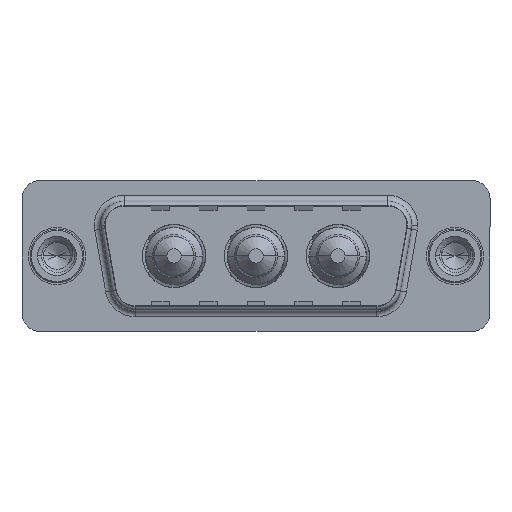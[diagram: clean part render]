
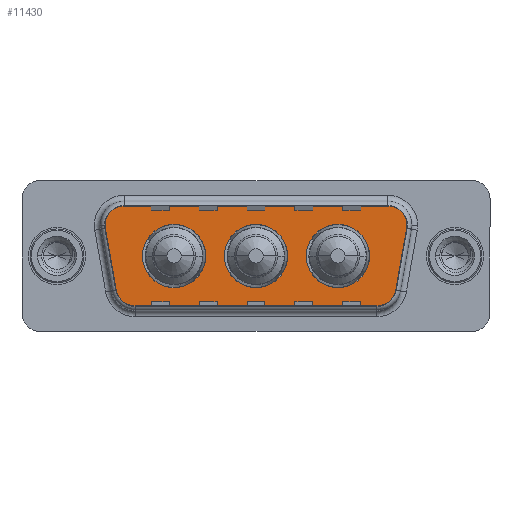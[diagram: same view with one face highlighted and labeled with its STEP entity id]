
A CAD part, top view. The second image highlights one B-rep face of the part: STEP entity #11430.
In plain terms, the highlighted planar face has unit normal (0, 0, 1).
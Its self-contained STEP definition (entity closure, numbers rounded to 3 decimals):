
#103 = VERTEX_POINT ( 'NONE', #378 ) ;
#166 = VERTEX_POINT ( 'NONE', #1659 ) ;
#203 = CARTESIAN_POINT ( 'NONE',  ( 16.65, 0., 0. ) ) ;
#204 = ORIENTED_EDGE ( 'NONE', *, *, #3101, .F. ) ;
#333 = CIRCLE ( 'NONE', #14607, 2.65 ) ;
#378 = CARTESIAN_POINT ( 'NONE',  ( 29.889, 2.9, 0. ) ) ;
#380 = VERTEX_POINT ( 'NONE', #7443 ) ;
#388 = LINE ( 'NONE', #12523, #9387 ) ;
#429 = AXIS2_PLACEMENT_3D ( 'NONE', #5937, #13932, #7087 ) ;
#430 = CIRCLE ( 'NONE', #7367, 2.65 ) ;
#561 = ORIENTED_EDGE ( 'NONE', *, *, #836, .F. ) ;
#836 = EDGE_CURVE ( 'NONE', #380, #11405, #6237, .T. ) ;
#867 = CIRCLE ( 'NONE', #3361, 2.65 ) ;
#938 = EDGE_CURVE ( 'NONE', #3575, #14402, #1811, .T. ) ;
#942 = CARTESIAN_POINT ( 'NONE',  ( 3.441, 2.553, 0. ) ) ;
#986 = CARTESIAN_POINT ( 'NONE',  ( 26.866, -2.9, 0. ) ) ;
#991 = DIRECTION ( 'NONE',  ( 0., 0., 1. ) ) ;
#1006 = CIRCLE ( 'NONE', #9244, 2.65 ) ;
#1277 = DIRECTION ( 'NONE',  ( 1., 0., 0. ) ) ;
#1309 = DIRECTION ( 'NONE',  ( 0.174, -0.985, 0. ) ) ;
#1363 = DIRECTION ( 'NONE',  ( 1., 0., 0. ) ) ;
#1579 = ORIENTED_EDGE ( 'NONE', *, *, #938, .T. ) ;
#1659 = CARTESIAN_POINT ( 'NONE',  ( 19.3, 0., 0. ) ) ;
#1811 = LINE ( 'NONE', #7647, #13191 ) ;
#2110 = DIRECTION ( 'NONE',  ( 0., 0., 1. ) ) ;
#2247 = EDGE_CURVE ( 'NONE', #9616, #3575, #11717, .T. ) ;
#2433 = VERTEX_POINT ( 'NONE', #6880 ) ;
#2488 = AXIS2_PLACEMENT_3D ( 'NONE', #986, #2110, #10003 ) ;
#2741 = ORIENTED_EDGE ( 'NONE', *, *, #8954, .T. ) ;
#2803 = CIRCLE ( 'NONE', #7224, 2. ) ;
#2817 = EDGE_LOOP ( 'NONE', ( #561, #14297 ) ) ;
#3101 = EDGE_CURVE ( 'NONE', #6075, #13467, #5824, .T. ) ;
#3361 = AXIS2_PLACEMENT_3D ( 'NONE', #203, #8092, #1363 ) ;
#3406 = CIRCLE ( 'NONE', #4661, 2. ) ;
#3575 = VERTEX_POINT ( 'NONE', #10072 ) ;
#3636 = DIRECTION ( 'NONE',  ( 0., 0., 1. ) ) ;
#3821 = ORIENTED_EDGE ( 'NONE', *, *, #10178, .T. ) ;
#3835 = CARTESIAN_POINT ( 'NONE',  ( 26.15, 0., 0. ) ) ;
#3862 = LINE ( 'NONE', #10329, #9684 ) ;
#3863 = CARTESIAN_POINT ( 'NONE',  ( 14., 0., 0. ) ) ;
#4349 = CARTESIAN_POINT ( 'NONE',  ( 7.15, 0., 0. ) ) ;
#4410 = EDGE_LOOP ( 'NONE', ( #204, #10141 ) ) ;
#4448 = EDGE_CURVE ( 'NONE', #12923, #7111, #2803, .T. ) ;
#4583 = DIRECTION ( 'NONE',  ( 0.174, 0.985, 0. ) ) ;
#4638 = DIRECTION ( 'NONE',  ( 0., 0., 1. ) ) ;
#4652 = CARTESIAN_POINT ( 'NONE',  ( 28.836, -3.247, 0. ) ) ;
#4661 = AXIS2_PLACEMENT_3D ( 'NONE', #11413, #4638, #12577 ) ;
#4729 = VERTEX_POINT ( 'NONE', #5823 ) ;
#4820 = DIRECTION ( 'NONE',  ( 0., 0., 1. ) ) ;
#5222 = ORIENTED_EDGE ( 'NONE', *, *, #4448, .T. ) ;
#5492 = ORIENTED_EDGE ( 'NONE', *, *, #12227, .F. ) ;
#5501 = LINE ( 'NONE', #13338, #8150 ) ;
#5823 = CARTESIAN_POINT ( 'NONE',  ( 29.859, 2.553, 0. ) ) ;
#5824 = CIRCLE ( 'NONE', #11785, 2.65 ) ;
#5937 = CARTESIAN_POINT ( 'NONE',  ( 27.889, 2.9, 0. ) ) ;
#6075 = VERTEX_POINT ( 'NONE', #3835 ) ;
#6237 = CIRCLE ( 'NONE', #6435, 2.65 ) ;
#6286 = VERTEX_POINT ( 'NONE', #3863 ) ;
#6430 = CIRCLE ( 'NONE', #9067, 2. ) ;
#6435 = AXIS2_PLACEMENT_3D ( 'NONE', #7254, #9954, #7124 ) ;
#6441 = CARTESIAN_POINT ( 'NONE',  ( 9.8, 0., 0. ) ) ;
#6507 = DIRECTION ( 'NONE',  ( -1., 0., 0. ) ) ;
#6655 = ORIENTED_EDGE ( 'NONE', *, *, #13512, .T. ) ;
#6880 = CARTESIAN_POINT ( 'NONE',  ( 27.889, 4.9, 0. ) ) ;
#6899 = FACE_BOUND ( 'NONE', #12753, .T. ) ;
#7061 = CARTESIAN_POINT ( 'NONE',  ( 4.464, -3.247, 0. ) ) ;
#7087 = DIRECTION ( 'NONE',  ( -1., 0., 0. ) ) ;
#7111 = VERTEX_POINT ( 'NONE', #942 ) ;
#7124 = DIRECTION ( 'NONE',  ( 1., 0., 0. ) ) ;
#7143 = EDGE_CURVE ( 'NONE', #6286, #166, #1006, .T. ) ;
#7224 = AXIS2_PLACEMENT_3D ( 'NONE', #11257, #11207, #11157 ) ;
#7254 = CARTESIAN_POINT ( 'NONE',  ( 9.8, 0., 0. ) ) ;
#7367 = AXIS2_PLACEMENT_3D ( 'NONE', #11610, #4820, #12775 ) ;
#7443 = CARTESIAN_POINT ( 'NONE',  ( 12.45, 0., 0. ) ) ;
#7564 = DIRECTION ( 'NONE',  ( 1., 0., 0. ) ) ;
#7647 = CARTESIAN_POINT ( 'NONE',  ( 6.434, -4.9, 0. ) ) ;
#7742 = PLANE ( 'NONE',  #2488 ) ;
#7745 = CARTESIAN_POINT ( 'NONE',  ( 16.65, 0., 0. ) ) ;
#8045 = AXIS2_PLACEMENT_3D ( 'NONE', #8888, #10400, #11605 ) ;
#8092 = DIRECTION ( 'NONE',  ( 0., 0., 1. ) ) ;
#8150 = VECTOR ( 'NONE', #6507, 1000. ) ;
#8243 = DIRECTION ( 'NONE',  ( 0., 0., 1. ) ) ;
#8264 = ORIENTED_EDGE ( 'NONE', *, *, #7143, .F. ) ;
#8442 = EDGE_CURVE ( 'NONE', #13467, #6075, #430, .T. ) ;
#8850 = DIRECTION ( 'NONE',  ( 1., 0., 0. ) ) ;
#8888 = CARTESIAN_POINT ( 'NONE',  ( 6.434, -2.9, 0. ) ) ;
#8954 = EDGE_CURVE ( 'NONE', #14402, #14713, #6430, .T. ) ;
#9067 = AXIS2_PLACEMENT_3D ( 'NONE', #10394, #3636, #11553 ) ;
#9244 = AXIS2_PLACEMENT_3D ( 'NONE', #7745, #991, #8850 ) ;
#9269 = CARTESIAN_POINT ( 'NONE',  ( 5.411, 4.9, 0. ) ) ;
#9387 = VECTOR ( 'NONE', #4583, 1000. ) ;
#9518 = FACE_OUTER_BOUND ( 'NONE', #12945, .T. ) ;
#9616 = VERTEX_POINT ( 'NONE', #7061 ) ;
#9684 = VECTOR ( 'NONE', #1309, 1000. ) ;
#9881 = FACE_BOUND ( 'NONE', #2817, .T. ) ;
#9921 = EDGE_CURVE ( 'NONE', #2433, #12923, #5501, .T. ) ;
#9954 = DIRECTION ( 'NONE',  ( 0., 0., 1. ) ) ;
#10003 = DIRECTION ( 'NONE',  ( 1., 0., 0. ) ) ;
#10072 = CARTESIAN_POINT ( 'NONE',  ( 6.434, -4.9, 0. ) ) ;
#10133 = EDGE_CURVE ( 'NONE', #14713, #4729, #388, .T. ) ;
#10141 = ORIENTED_EDGE ( 'NONE', *, *, #8442, .F. ) ;
#10178 = EDGE_CURVE ( 'NONE', #4729, #103, #3406, .T. ) ;
#10286 = ORIENTED_EDGE ( 'NONE', *, *, #10133, .T. ) ;
#10329 = CARTESIAN_POINT ( 'NONE',  ( 3.441, 2.553, 0. ) ) ;
#10394 = CARTESIAN_POINT ( 'NONE',  ( 26.866, -2.9, 0. ) ) ;
#10400 = DIRECTION ( 'NONE',  ( 0., 0., 1. ) ) ;
#10459 = ORIENTED_EDGE ( 'NONE', *, *, #2247, .T. ) ;
#11157 = DIRECTION ( 'NONE',  ( 1., 0., 0. ) ) ;
#11207 = DIRECTION ( 'NONE',  ( 0., 0., 1. ) ) ;
#11257 = CARTESIAN_POINT ( 'NONE',  ( 5.411, 2.9, 0. ) ) ;
#11304 = DIRECTION ( 'NONE',  ( 1., 0., 0. ) ) ;
#11344 = ORIENTED_EDGE ( 'NONE', *, *, #9921, .T. ) ;
#11405 = VERTEX_POINT ( 'NONE', #4349 ) ;
#11413 = CARTESIAN_POINT ( 'NONE',  ( 27.889, 2.9, 0. ) ) ;
#11430 = ADVANCED_FACE ( 'NONE', ( #6899, #12604, #9881, #9518 ), #7742, .T. ) ;
#11553 = DIRECTION ( 'NONE',  ( 1., 0., 0. ) ) ;
#11605 = DIRECTION ( 'NONE',  ( -1., 0., 0. ) ) ;
#11610 = CARTESIAN_POINT ( 'NONE',  ( 23.5, 0., 0. ) ) ;
#11717 = CIRCLE ( 'NONE', #8045, 2. ) ;
#11785 = AXIS2_PLACEMENT_3D ( 'NONE', #14525, #8243, #11304 ) ;
#11936 = EDGE_CURVE ( 'NONE', #11405, #380, #333, .T. ) ;
#12221 = EDGE_CURVE ( 'NONE', #7111, #9616, #3862, .T. ) ;
#12227 = EDGE_CURVE ( 'NONE', #166, #6286, #867, .T. ) ;
#12523 = CARTESIAN_POINT ( 'NONE',  ( 29.859, 2.553, 0. ) ) ;
#12577 = DIRECTION ( 'NONE',  ( -1., 0., 0. ) ) ;
#12604 = FACE_BOUND ( 'NONE', #4410, .T. ) ;
#12753 = EDGE_LOOP ( 'NONE', ( #5492, #8264 ) ) ;
#12775 = DIRECTION ( 'NONE',  ( 1., 0., 0. ) ) ;
#12923 = VERTEX_POINT ( 'NONE', #9269 ) ;
#12945 = EDGE_LOOP ( 'NONE', ( #2741, #10286, #3821, #6655, #11344, #5222, #14018, #10459, #1579 ) ) ;
#13191 = VECTOR ( 'NONE', #1277, 1000. ) ;
#13197 = CARTESIAN_POINT ( 'NONE',  ( 26.866, -4.9, 0. ) ) ;
#13338 = CARTESIAN_POINT ( 'NONE',  ( 5.411, 4.9, 0. ) ) ;
#13467 = VERTEX_POINT ( 'NONE', #13737 ) ;
#13512 = EDGE_CURVE ( 'NONE', #103, #2433, #14007, .T. ) ;
#13737 = CARTESIAN_POINT ( 'NONE',  ( 20.85, 0., 0. ) ) ;
#13932 = DIRECTION ( 'NONE',  ( 0., 0., 1. ) ) ;
#14007 = CIRCLE ( 'NONE', #429, 2. ) ;
#14018 = ORIENTED_EDGE ( 'NONE', *, *, #12221, .T. ) ;
#14297 = ORIENTED_EDGE ( 'NONE', *, *, #11936, .F. ) ;
#14402 = VERTEX_POINT ( 'NONE', #13197 ) ;
#14439 = DIRECTION ( 'NONE',  ( 0., 0., 1. ) ) ;
#14525 = CARTESIAN_POINT ( 'NONE',  ( 23.5, 0., 0. ) ) ;
#14607 = AXIS2_PLACEMENT_3D ( 'NONE', #6441, #14439, #7564 ) ;
#14713 = VERTEX_POINT ( 'NONE', #4652 ) ;
